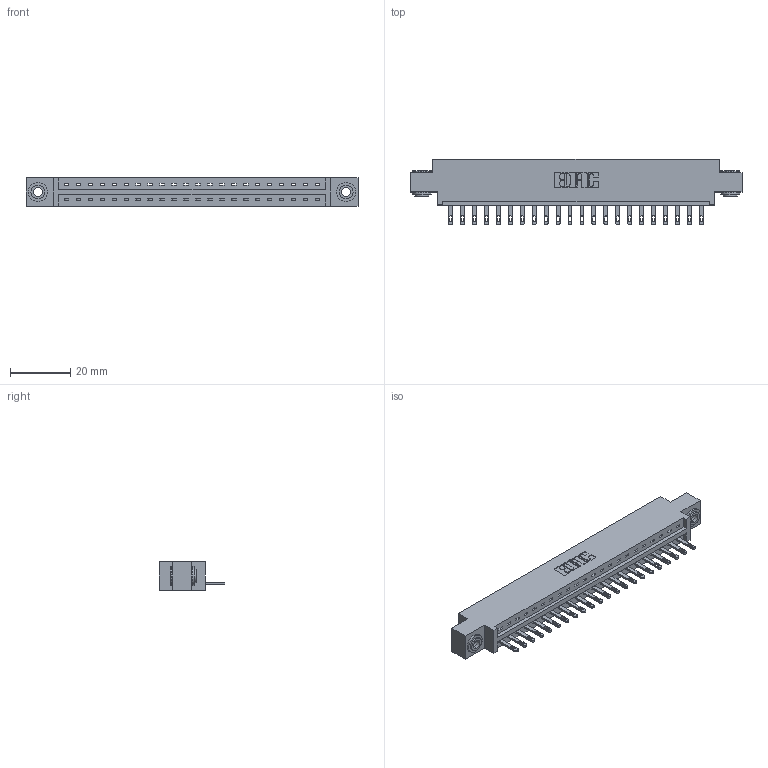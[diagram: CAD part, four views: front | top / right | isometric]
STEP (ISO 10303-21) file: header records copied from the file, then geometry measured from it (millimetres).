
FILE_DESCRIPTION (( 'STEP AP203' ), '1' );
FILE_NAME ('887-022-500-603.STEP', '2020-09-20T18:40:00', ( '' ), ( '' ), 'SwSTEP 2.0', 'SolidWorks 2020', '' );
FILE_SCHEMA (( 'CONFIG_CONTROL_DESIGN' ));
Length unit declared in the file: inch
Products named in the file (4): 345-292-001_345-293-100; 887-022-500-603; 345-250-002_345-250-002-102; 837 Part_0.170 Offset - 0.156 Dia-TH
Assembly tree (25 placements, depth 2):
  887-022-500-603
    837 Part_0.170 Offset - 0.156 Dia-TH
    345-292-001_345-293-100  x22
    345-250-002_345-250-002-102  x2
Bounding box: 110.19 x 21.85 x 9.4 mm (x, y, z)
Volume: 11117.1 mm3; surface area: 11757.4 mm2
Topology: 25 solids, 25 shells, 1432 faces, 4359 edges, 2902 vertices
Faces by surface type: plane 964, cylinder 460, cone 8
Entity records: 19652 total; most frequent: CARTESIAN_POINT 3399, ORIENTED_EDGE 3350, DIRECTION 2937, EDGE_CURVE 1675, LINE 1519, VECTOR 1519, VERTEX_POINT 1114, AXIS2_PLACEMENT_3D 709
